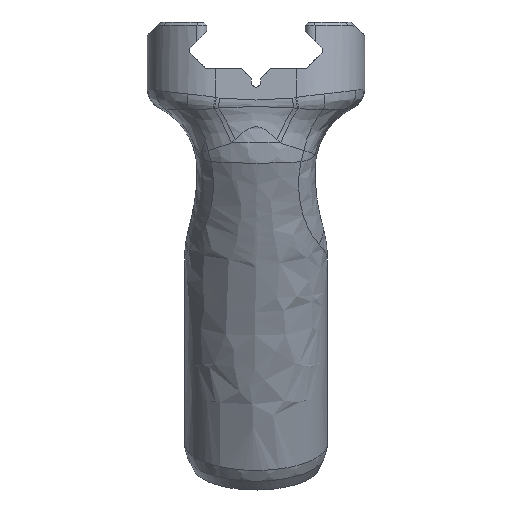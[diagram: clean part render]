
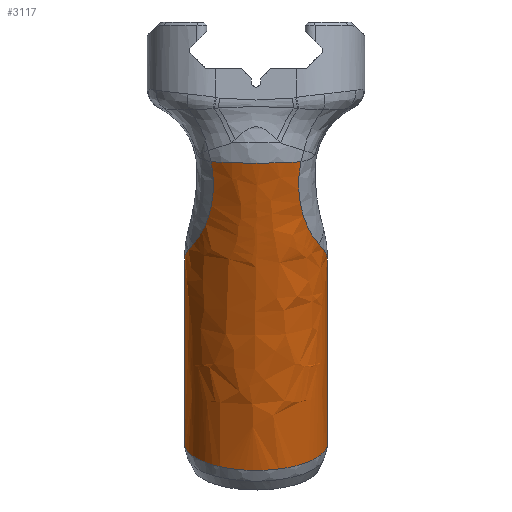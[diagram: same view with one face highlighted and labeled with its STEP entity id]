
A CAD part, front view. The second image highlights one B-rep face of the part: STEP entity #3117.
In plain terms, the highlighted free-form (B-spline) face has degree [1, 2] with [2, 5] control points.
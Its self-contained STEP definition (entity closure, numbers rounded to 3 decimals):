
#16=(
BOUNDED_SURFACE()
B_SPLINE_SURFACE(1,2,((#6084,#6085,#6086,#6087,#6088),(#6089,#6090,#6091,
#6092,#6093)),.UNSPECIFIED.,.F.,.F.,.F.)
B_SPLINE_SURFACE_WITH_KNOTS((2,2),(3,2,3),(0.251,4.977),
(0.,1.571,3.142),.UNSPECIFIED.)
GEOMETRIC_REPRESENTATION_ITEM()
RATIONAL_B_SPLINE_SURFACE(((1.,0.707,1.,0.707,1.),
(1.,0.707,1.,0.707,1.)))
REPRESENTATION_ITEM('')
SURFACE()
);
#264=B_SPLINE_CURVE_WITH_KNOTS('',3,(#5919,#5920,#5921,#5922,#5923,#5924,
#5925,#5926,#5927,#5928,#5929,#5930),.UNSPECIFIED.,.F.,.F.,(4,1,1,1,1,1,
1,1,1,4),(0.,0.134,0.269,0.537,0.806,
1.075,1.343,1.612,1.747,1.881),
 .UNSPECIFIED.);
#272=B_SPLINE_CURVE_WITH_KNOTS('',3,(#6097,#6098,#6099,#6100,#6101,#6102),
 .UNSPECIFIED.,.F.,.F.,(4,2,4),(-0.549,0.,0.002),
 .UNSPECIFIED.);
#273=B_SPLINE_CURVE_WITH_KNOTS('',3,(#6104,#6105,#6106,#6107,#6108,#6109,
#6110),.UNSPECIFIED.,.F.,.F.,(4,1,1,1,4),(-1.623,-1.159,
-0.696,-0.232,0.),.UNSPECIFIED.);
#274=B_SPLINE_CURVE_WITH_KNOTS('',3,(#6112,#6113,#6114,#6115,#6116,#6117,
#6118),.UNSPECIFIED.,.F.,.F.,(4,1,1,1,4),(-0.861,-0.781,
-0.621,-0.461,-0.301),.UNSPECIFIED.);
#275=B_SPLINE_CURVE_WITH_KNOTS('',3,(#6120,#6121,#6122,#6123,#6124,#6125,
#6126,#6127),.UNSPECIFIED.,.F.,.F.,(4,1,1,1,1,4),(-1.623,-1.391,
-1.159,-0.928,-0.464,0.),
 .UNSPECIFIED.);
#276=B_SPLINE_CURVE_WITH_KNOTS('',3,(#6128,#6129,#6130,#6131,#6132,#6133),
 .UNSPECIFIED.,.F.,.F.,(4,2,4),(-0.551,-0.549,0.),
 .UNSPECIFIED.);
#568=FACE_OUTER_BOUND('',#770,.T.);
#770=EDGE_LOOP('',(#2405,#2406,#2407,#2408,#2409,#2410,#2411,#2412));
#982=LINE('',#6040,#1127);
#985=LINE('',#6095,#1130);
#1127=VECTOR('',#3795,10.);
#1130=VECTOR('',#3800,10.);
#1379=VERTEX_POINT('',#5771);
#1384=VERTEX_POINT('',#5854);
#1394=VERTEX_POINT('',#6039);
#1395=VERTEX_POINT('',#6094);
#1396=VERTEX_POINT('',#6096);
#1397=VERTEX_POINT('',#6103);
#1398=VERTEX_POINT('',#6111);
#1399=VERTEX_POINT('',#6119);
#1752=EDGE_CURVE('',#1384,#1379,#264,.T.);
#1765=EDGE_CURVE('',#1379,#1394,#982,.T.);
#1768=EDGE_CURVE('',#1384,#1395,#985,.T.);
#1769=EDGE_CURVE('',#1396,#1395,#272,.T.);
#1770=EDGE_CURVE('',#1397,#1396,#273,.T.);
#1771=EDGE_CURVE('',#1398,#1397,#274,.T.);
#1772=EDGE_CURVE('',#1399,#1398,#275,.T.);
#1773=EDGE_CURVE('',#1394,#1399,#276,.T.);
#2405=ORIENTED_EDGE('',*,*,#1752,.F.);
#2406=ORIENTED_EDGE('',*,*,#1768,.T.);
#2407=ORIENTED_EDGE('',*,*,#1769,.F.);
#2408=ORIENTED_EDGE('',*,*,#1770,.F.);
#2409=ORIENTED_EDGE('',*,*,#1771,.F.);
#2410=ORIENTED_EDGE('',*,*,#1772,.F.);
#2411=ORIENTED_EDGE('',*,*,#1773,.F.);
#2412=ORIENTED_EDGE('',*,*,#1765,.F.);
#3117=ADVANCED_FACE('',(#568),#16,.F.);
#3795=DIRECTION('',(0.,-0.415,0.91));
#3800=DIRECTION('',(0.,-0.415,0.91));
#5771=CARTESIAN_POINT('',(-11.5,65.814,-73.898));
#5854=CARTESIAN_POINT('',(11.5,65.814,-73.898));
#5919=CARTESIAN_POINT('Ctrl Pts',(11.5,65.814,-73.898));
#5920=CARTESIAN_POINT('Ctrl Pts',(11.5,64.956,-74.29));
#5921=CARTESIAN_POINT('Ctrl Pts',(11.214,63.243,-75.072));
#5922=CARTESIAN_POINT('Ctrl Pts',(9.659,60.247,-76.439));
#5923=CARTESIAN_POINT('Ctrl Pts',(6.563,57.664,-77.618));
#5924=CARTESIAN_POINT('Ctrl Pts',(2.243,56.237,-78.269));
#5925=CARTESIAN_POINT('Ctrl Pts',(-2.244,56.238,-78.269));
#5926=CARTESIAN_POINT('Ctrl Pts',(-6.569,57.665,-77.617));
#5927=CARTESIAN_POINT('Ctrl Pts',(-9.657,60.245,-76.44));
#5928=CARTESIAN_POINT('Ctrl Pts',(-11.213,63.243,-75.072));
#5929=CARTESIAN_POINT('Ctrl Pts',(-11.5,64.956,-74.29));
#5930=CARTESIAN_POINT('Ctrl Pts',(-11.5,65.814,-73.898));
#6039=CARTESIAN_POINT('',(-11.5,52.347,-44.39));
#6040=CARTESIAN_POINT('',(-11.5,67.011,-76.521));
#6084=CARTESIAN_POINT('Ctrl Pts',(-11.5,65.814,-73.898));
#6085=CARTESIAN_POINT('Ctrl Pts',(-11.5,56.296,-78.242));
#6086=CARTESIAN_POINT('Ctrl Pts',(0.,56.296,
-78.242));
#6087=CARTESIAN_POINT('Ctrl Pts',(11.5,56.296,-78.242));
#6088=CARTESIAN_POINT('Ctrl Pts',(11.5,65.814,-73.898));
#6089=CARTESIAN_POINT('Ctrl Pts',(-11.5,43.247,-24.451));
#6090=CARTESIAN_POINT('Ctrl Pts',(-11.5,33.73,-28.795));
#6091=CARTESIAN_POINT('Ctrl Pts',(0.,33.73,
-28.795));
#6092=CARTESIAN_POINT('Ctrl Pts',(11.5,33.73,-28.795));
#6093=CARTESIAN_POINT('Ctrl Pts',(11.5,43.247,-24.451));
#6094=CARTESIAN_POINT('',(11.5,52.347,-44.39));
#6095=CARTESIAN_POINT('',(11.5,67.011,-76.521));
#6096=CARTESIAN_POINT('',(10.105,45.672,-41.794));
#6097=CARTESIAN_POINT('Ctrl Pts',(10.105,45.672,-41.794));
#6098=CARTESIAN_POINT('Ctrl Pts',(10.998,47.732,-42.707));
#6099=CARTESIAN_POINT('Ctrl Pts',(11.498,50.018,-43.55));
#6100=CARTESIAN_POINT('Ctrl Pts',(11.5,52.332,-44.384));
#6101=CARTESIAN_POINT('Ctrl Pts',(11.5,52.339,-44.387));
#6102=CARTESIAN_POINT('Ctrl Pts',(11.5,52.347,-44.39));
#6103=CARTESIAN_POINT('',(7.238,36.191,-28.571));
#6104=CARTESIAN_POINT('Ctrl Pts',(7.238,36.191,-28.571));
#6105=CARTESIAN_POINT('Ctrl Pts',(6.938,36.628,-30.06));
#6106=CARTESIAN_POINT('Ctrl Pts',(6.709,37.78,-32.937));
#6107=CARTESIAN_POINT('Ctrl Pts',(7.344,40.087,-36.974));
#6108=CARTESIAN_POINT('Ctrl Pts',(8.646,42.634,-39.984));
#6109=CARTESIAN_POINT('Ctrl Pts',(9.728,44.803,-41.409));
#6110=CARTESIAN_POINT('Ctrl Pts',(10.105,45.672,-41.794));
#6111=CARTESIAN_POINT('',(-7.238,36.191,-28.571));
#6112=CARTESIAN_POINT('Ctrl Pts',(-7.238,36.191,-28.571));
#6113=CARTESIAN_POINT('Ctrl Pts',(-6.632,35.723,-28.621));
#6114=CARTESIAN_POINT('Ctrl Pts',(-4.707,34.52,-28.736));
#6115=CARTESIAN_POINT('Ctrl Pts',(-1.114,33.509,-28.81));
#6116=CARTESIAN_POINT('Ctrl Pts',(3.312,33.914,-28.783));
#6117=CARTESIAN_POINT('Ctrl Pts',(6.026,35.255,-28.671));
#6118=CARTESIAN_POINT('Ctrl Pts',(7.238,36.191,-28.571));
#6119=CARTESIAN_POINT('',(-10.105,45.672,-41.794));
#6120=CARTESIAN_POINT('Ctrl Pts',(-10.105,45.672,-41.794));
#6121=CARTESIAN_POINT('Ctrl Pts',(-9.728,44.803,-41.409));
#6122=CARTESIAN_POINT('Ctrl Pts',(-9.007,43.351,-40.462));
#6123=CARTESIAN_POINT('Ctrl Pts',(-8.124,41.621,-38.777));
#6124=CARTESIAN_POINT('Ctrl Pts',(-7.239,39.698,-36.304));
#6125=CARTESIAN_POINT('Ctrl Pts',(-6.709,37.784,-32.935));
#6126=CARTESIAN_POINT('Ctrl Pts',(-6.938,36.628,-30.06));
#6127=CARTESIAN_POINT('Ctrl Pts',(-7.238,36.191,-28.571));
#6128=CARTESIAN_POINT('Ctrl Pts',(-11.5,52.347,-44.39));
#6129=CARTESIAN_POINT('Ctrl Pts',(-11.5,52.339,-44.387));
#6130=CARTESIAN_POINT('Ctrl Pts',(-11.5,52.332,-44.384));
#6131=CARTESIAN_POINT('Ctrl Pts',(-11.498,50.017,-43.55));
#6132=CARTESIAN_POINT('Ctrl Pts',(-10.998,47.732,-42.707));
#6133=CARTESIAN_POINT('Ctrl Pts',(-10.105,45.672,-41.794));
